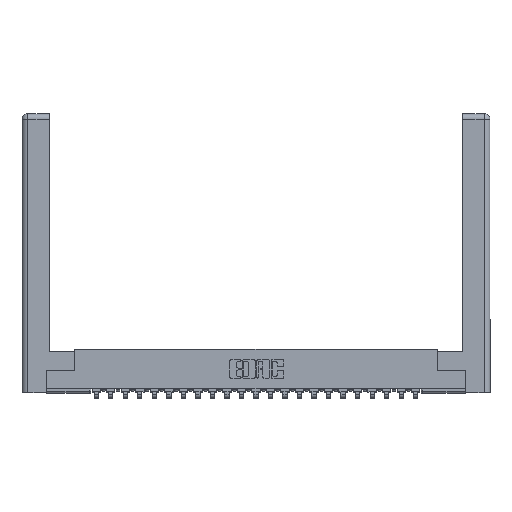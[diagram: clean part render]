
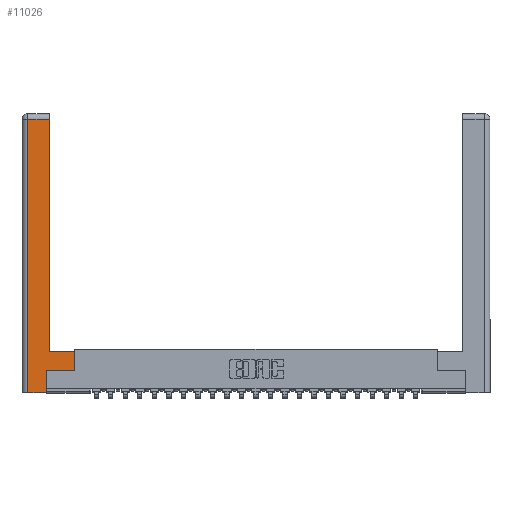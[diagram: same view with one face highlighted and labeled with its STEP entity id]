
A CAD part, top view. The second image highlights one B-rep face of the part: STEP entity #11026.
In plain terms, the highlighted planar face has unit normal (0, 0, 1).
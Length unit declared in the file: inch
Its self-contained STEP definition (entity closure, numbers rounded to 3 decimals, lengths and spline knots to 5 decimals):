
#643 = LINE ( 'NONE', #12426, #8618 ) ;
#974 = VECTOR ( 'NONE', #19054, 39.37008 ) ;
#1076 = EDGE_CURVE ( 'NONE', #11636, #8998, #7153, .T. ) ;
#1470 = EDGE_CURVE ( 'NONE', #24820, #11636, #643, .T. ) ;
#1523 = FACE_OUTER_BOUND ( 'NONE', #6901, .T. ) ;
#1719 = CARTESIAN_POINT ( 'NONE',  ( 0.565, 0.245, 0. ) ) ;
#2106 = CARTESIAN_POINT ( 'NONE',  ( 0.265, 0.245, 0. ) ) ;
#2776 = VERTEX_POINT ( 'NONE', #16262 ) ;
#2960 = VECTOR ( 'NONE', #22741, 39.37008 ) ;
#2989 = LINE ( 'NONE', #18864, #23326 ) ;
#3354 = ORIENTED_EDGE ( 'NONE', *, *, #1470, .T. ) ;
#3415 = VECTOR ( 'NONE', #8123, 39.37008 ) ;
#3854 = VECTOR ( 'NONE', #25466, 39.37008 ) ;
#4699 = CARTESIAN_POINT ( 'NONE',  ( 0.265, 0., 0. ) ) ;
#4761 = DIRECTION ( 'NONE',  ( 1., 0., 0. ) ) ;
#5755 = CARTESIAN_POINT ( 'NONE',  ( 0.0615, 2.94, 0. ) ) ;
#5979 = CARTESIAN_POINT ( 'NONE',  ( 0.565, 0.45, 0. ) ) ;
#6901 = EDGE_LOOP ( 'NONE', ( #9953, #19315, #21701, #9566, #13670, #3354, #11808, #25070 ) ) ;
#6915 = LINE ( 'NONE', #5755, #3854 ) ;
#7038 = DIRECTION ( 'NONE',  ( -1., 0., 0. ) ) ;
#7153 = LINE ( 'NONE', #8543, #20349 ) ;
#7486 = CARTESIAN_POINT ( 'NONE',  ( 0.0615, 2.94, 0. ) ) ;
#7528 = DIRECTION ( 'NONE',  ( -1., 0., 0. ) ) ;
#7945 = EDGE_CURVE ( 'NONE', #2776, #17633, #13613, .T. ) ;
#8123 = DIRECTION ( 'NONE',  ( 0., 1., 0. ) ) ;
#8543 = CARTESIAN_POINT ( 'NONE',  ( 0.565, 0.45, 0. ) ) ;
#8618 = VECTOR ( 'NONE', #4761, 39.37008 ) ;
#8691 = CARTESIAN_POINT ( 'NONE',  ( 0.295, 2.94, 0. ) ) ;
#8998 = VERTEX_POINT ( 'NONE', #5979 ) ;
#9566 = ORIENTED_EDGE ( 'NONE', *, *, #18741, .T. ) ;
#9767 = EDGE_CURVE ( 'NONE', #16626, #22424, #11073, .T. ) ;
#9953 = ORIENTED_EDGE ( 'NONE', *, *, #7945, .T. ) ;
#10239 = VECTOR ( 'NONE', #11970, 39.37008 ) ;
#10511 = EDGE_CURVE ( 'NONE', #19509, #24820, #23742, .T. ) ;
#10875 = CARTESIAN_POINT ( 'NONE',  ( 0.0615, 0., 0. ) ) ;
#11026 = ADVANCED_FACE ( 'NONE', ( #1523 ), #15545, .F. ) ;
#11073 = LINE ( 'NONE', #10875, #974 ) ;
#11636 = VERTEX_POINT ( 'NONE', #1719 ) ;
#11808 = ORIENTED_EDGE ( 'NONE', *, *, #1076, .T. ) ;
#11970 = DIRECTION ( 'NONE',  ( 0., 1., 0. ) ) ;
#12426 = CARTESIAN_POINT ( 'NONE',  ( 0.565, 0.245, 0. ) ) ;
#12463 = DIRECTION ( 'NONE',  ( 0., 1., 0. ) ) ;
#13613 = LINE ( 'NONE', #23849, #10239 ) ;
#13670 = ORIENTED_EDGE ( 'NONE', *, *, #10511, .T. ) ;
#14727 = EDGE_CURVE ( 'NONE', #8998, #2776, #2989, .T. ) ;
#15545 = PLANE ( 'NONE',  #24915 ) ;
#16262 = CARTESIAN_POINT ( 'NONE',  ( 0.295, 0.45, 0. ) ) ;
#16626 = VERTEX_POINT ( 'NONE', #7486 ) ;
#17531 = DIRECTION ( 'NONE',  ( 0., 0., -1. ) ) ;
#17617 = CARTESIAN_POINT ( 'NONE',  ( 0., 0., 0. ) ) ;
#17633 = VERTEX_POINT ( 'NONE', #8691 ) ;
#18374 = CARTESIAN_POINT ( 'NONE',  ( 0.0615, 0., 0. ) ) ;
#18607 = LINE ( 'NONE', #4699, #2960 ) ;
#18741 = EDGE_CURVE ( 'NONE', #22424, #19509, #18607, .T. ) ;
#18864 = CARTESIAN_POINT ( 'NONE',  ( 0.295, 0.45, 0. ) ) ;
#19054 = DIRECTION ( 'NONE',  ( 0., -1., 0. ) ) ;
#19315 = ORIENTED_EDGE ( 'NONE', *, *, #20271, .T. ) ;
#19509 = VERTEX_POINT ( 'NONE', #24911 ) ;
#20271 = EDGE_CURVE ( 'NONE', #17633, #16626, #6915, .T. ) ;
#20349 = VECTOR ( 'NONE', #12463, 39.37008 ) ;
#21546 = CARTESIAN_POINT ( 'NONE',  ( 0.265, 0.245, 0. ) ) ;
#21701 = ORIENTED_EDGE ( 'NONE', *, *, #9767, .T. ) ;
#22424 = VERTEX_POINT ( 'NONE', #18374 ) ;
#22741 = DIRECTION ( 'NONE',  ( 1., 0., 0. ) ) ;
#23326 = VECTOR ( 'NONE', #7038, 39.37008 ) ;
#23742 = LINE ( 'NONE', #21546, #3415 ) ;
#23849 = CARTESIAN_POINT ( 'NONE',  ( 0.295, 3., 0. ) ) ;
#24820 = VERTEX_POINT ( 'NONE', #2106 ) ;
#24911 = CARTESIAN_POINT ( 'NONE',  ( 0.265, 0., 0. ) ) ;
#24915 = AXIS2_PLACEMENT_3D ( 'NONE', #17617, #17531, #7528 ) ;
#25070 = ORIENTED_EDGE ( 'NONE', *, *, #14727, .T. ) ;
#25466 = DIRECTION ( 'NONE',  ( -1., 0., 0. ) ) ;
